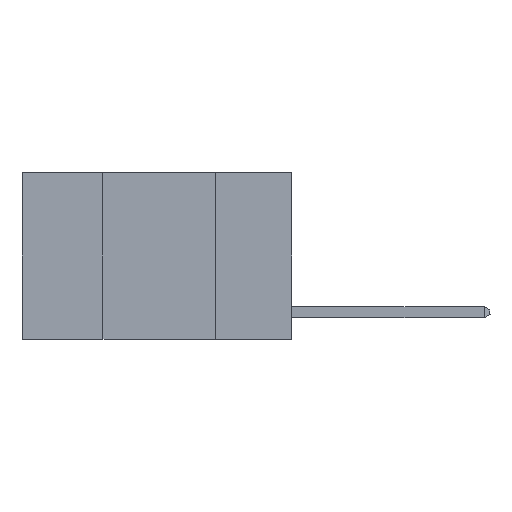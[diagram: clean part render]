
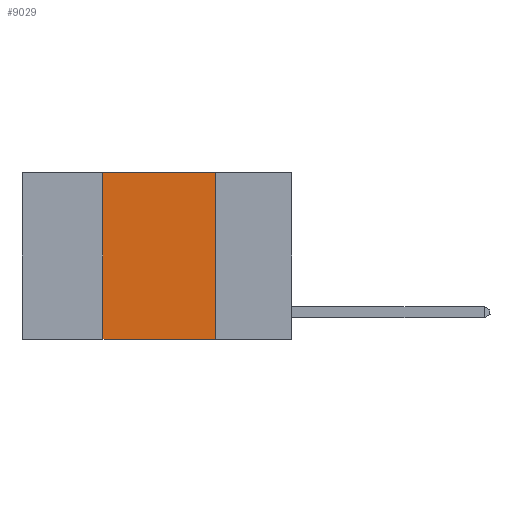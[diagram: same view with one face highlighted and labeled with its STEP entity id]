
A CAD part, left-side view. The second image highlights one B-rep face of the part: STEP entity #9029.
In plain terms, the highlighted planar face has unit normal (-1, 0, 0).
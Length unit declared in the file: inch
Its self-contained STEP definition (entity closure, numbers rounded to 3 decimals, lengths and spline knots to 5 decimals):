
#69 = CARTESIAN_POINT ( 'NONE',  ( 0., 0.42, -0.37 ) ) ;
#462 = VERTEX_POINT ( 'NONE', #659 ) ;
#659 = CARTESIAN_POINT ( 'NONE',  ( 0., 0.42, 0. ) ) ;
#704 = VECTOR ( 'NONE', #9816, 39.37008 ) ;
#886 = CARTESIAN_POINT ( 'NONE',  ( 0., 0.42, 0. ) ) ;
#1303 = CARTESIAN_POINT ( 'NONE',  ( 0., 0.6, 0. ) ) ;
#1522 = VECTOR ( 'NONE', #12120, 39.37008 ) ;
#1793 = VERTEX_POINT ( 'NONE', #69 ) ;
#2128 = EDGE_CURVE ( 'NONE', #1793, #8217, #8111, .T. ) ;
#2363 = CARTESIAN_POINT ( 'NONE',  ( 0., 0.6, 0. ) ) ;
#3028 = EDGE_CURVE ( 'NONE', #3618, #8217, #4203, .T. ) ;
#3608 = CARTESIAN_POINT ( 'NONE',  ( 0., 0.17, -0.37 ) ) ;
#3618 = VERTEX_POINT ( 'NONE', #9936 ) ;
#3891 = ORIENTED_EDGE ( 'NONE', *, *, #2128, .T. ) ;
#4015 = AXIS2_PLACEMENT_3D ( 'NONE', #2363, #9070, #13417 ) ;
#4203 = LINE ( 'NONE', #5182, #704 ) ;
#4549 = EDGE_CURVE ( 'NONE', #462, #3618, #13058, .T. ) ;
#4768 = PLANE ( 'NONE',  #4015 ) ;
#5048 = LINE ( 'NONE', #886, #10202 ) ;
#5182 = CARTESIAN_POINT ( 'NONE',  ( 0., 0.17, 0. ) ) ;
#5592 = FACE_OUTER_BOUND ( 'NONE', #8325, .T. ) ;
#5678 = EDGE_CURVE ( 'NONE', #1793, #462, #5048, .T. ) ;
#5973 = DIRECTION ( 'NONE',  ( 0., -1., 0. ) ) ;
#8111 = LINE ( 'NONE', #11560, #12947 ) ;
#8217 = VERTEX_POINT ( 'NONE', #3608 ) ;
#8325 = EDGE_LOOP ( 'NONE', ( #12766, #10891, #12650, #3891 ) ) ;
#9029 = ADVANCED_FACE ( 'NONE', ( #5592 ), #4768, .F. ) ;
#9070 = DIRECTION ( 'NONE',  ( 1., 0., 0. ) ) ;
#9816 = DIRECTION ( 'NONE',  ( 0., 0., -1. ) ) ;
#9936 = CARTESIAN_POINT ( 'NONE',  ( 0., 0.17, 0. ) ) ;
#10202 = VECTOR ( 'NONE', #13929, 39.37008 ) ;
#10891 = ORIENTED_EDGE ( 'NONE', *, *, #4549, .F. ) ;
#11560 = CARTESIAN_POINT ( 'NONE',  ( 0., 0.6, -0.37 ) ) ;
#12120 = DIRECTION ( 'NONE',  ( 0., -1., 0. ) ) ;
#12650 = ORIENTED_EDGE ( 'NONE', *, *, #5678, .F. ) ;
#12766 = ORIENTED_EDGE ( 'NONE', *, *, #3028, .F. ) ;
#12947 = VECTOR ( 'NONE', #5973, 39.37008 ) ;
#13058 = LINE ( 'NONE', #1303, #1522 ) ;
#13417 = DIRECTION ( 'NONE',  ( 0., 0., -1. ) ) ;
#13929 = DIRECTION ( 'NONE',  ( 0., 0., 1. ) ) ;
